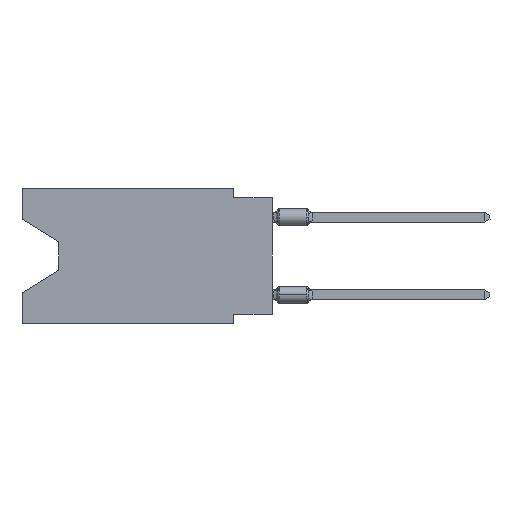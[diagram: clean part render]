
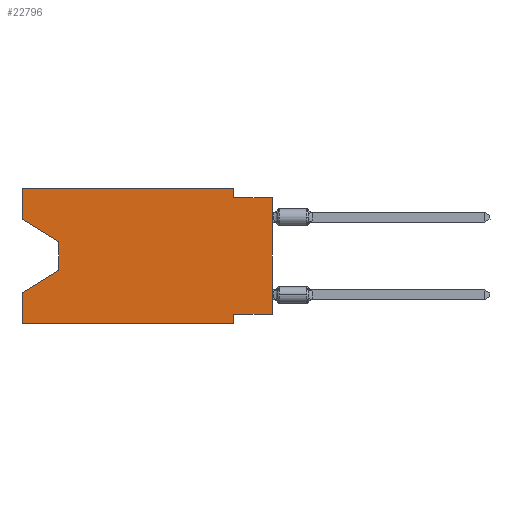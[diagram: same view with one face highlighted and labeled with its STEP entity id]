
A CAD part, left-side view. The second image highlights one B-rep face of the part: STEP entity #22796.
In plain terms, the highlighted planar face has unit normal (-1, 0, 0).
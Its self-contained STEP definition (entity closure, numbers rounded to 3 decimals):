
#113 = CARTESIAN_POINT ( 'NONE',  ( 0., 16.383, 0. ) ) ;
#532 = VERTEX_POINT ( 'NONE', #19451 ) ;
#1204 = EDGE_CURVE ( 'NONE', #12991, #24215, #21346, .T. ) ;
#1276 = VECTOR ( 'NONE', #21200, 1000. ) ;
#1779 = CARTESIAN_POINT ( 'NONE',  ( 0., 16.383, -8.89 ) ) ;
#1817 = CARTESIAN_POINT ( 'NONE',  ( 0., 13.97, -3.505 ) ) ;
#2605 = LINE ( 'NONE', #20838, #26267 ) ;
#3109 = VERTEX_POINT ( 'NONE', #23534 ) ;
#3121 = VERTEX_POINT ( 'NONE', #30328 ) ;
#3627 = EDGE_CURVE ( 'NONE', #6802, #29705, #21899, .T. ) ;
#3643 = CARTESIAN_POINT ( 'NONE',  ( 0., 16.383, -6.852 ) ) ;
#3694 = VECTOR ( 'NONE', #18195, 1000. ) ;
#3832 = LINE ( 'NONE', #1817, #3694 ) ;
#4683 = CARTESIAN_POINT ( 'NONE',  ( 0., 0., 0. ) ) ;
#4834 = VECTOR ( 'NONE', #29973, 1000. ) ;
#5129 = VERTEX_POINT ( 'NONE', #8794 ) ;
#5276 = CARTESIAN_POINT ( 'NONE',  ( 0., 0., -8.255 ) ) ;
#6111 = FACE_OUTER_BOUND ( 'NONE', #15059, .T. ) ;
#6137 = CARTESIAN_POINT ( 'NONE',  ( 0., 13.97, -5.385 ) ) ;
#6257 = VECTOR ( 'NONE', #30333, 1000. ) ;
#6549 = VERTEX_POINT ( 'NONE', #25130 ) ;
#6802 = VERTEX_POINT ( 'NONE', #9281 ) ;
#7530 = DIRECTION ( 'NONE',  ( 0., 0., -1. ) ) ;
#7658 = VERTEX_POINT ( 'NONE', #25699 ) ;
#8290 = DIRECTION ( 'NONE',  ( 0., 0.855, -0.519 ) ) ;
#8420 = EDGE_CURVE ( 'NONE', #3109, #6549, #2605, .T. ) ;
#8794 = CARTESIAN_POINT ( 'NONE',  ( 0., 0., -0.635 ) ) ;
#9281 = CARTESIAN_POINT ( 'NONE',  ( 0., 2.54, 0. ) ) ;
#9352 = ORIENTED_EDGE ( 'NONE', *, *, #14881, .F. ) ;
#9777 = ORIENTED_EDGE ( 'NONE', *, *, #25870, .T. ) ;
#10155 = CARTESIAN_POINT ( 'NONE',  ( 0., 2.54, 0. ) ) ;
#10588 = CARTESIAN_POINT ( 'NONE',  ( 0., 16.383, 0. ) ) ;
#11511 = ORIENTED_EDGE ( 'NONE', *, *, #15652, .T. ) ;
#12054 = LINE ( 'NONE', #20872, #18426 ) ;
#12399 = LINE ( 'NONE', #23833, #14665 ) ;
#12660 = EDGE_CURVE ( 'NONE', #13070, #26617, #17886, .T. ) ;
#12991 = VERTEX_POINT ( 'NONE', #22790 ) ;
#13070 = VERTEX_POINT ( 'NONE', #1779 ) ;
#13263 = CARTESIAN_POINT ( 'NONE',  ( 0., 16.383, 0. ) ) ;
#13536 = PLANE ( 'NONE',  #21171 ) ;
#14126 = CARTESIAN_POINT ( 'NONE',  ( 0., 16.383, 0. ) ) ;
#14665 = VECTOR ( 'NONE', #14713, 1000. ) ;
#14713 = DIRECTION ( 'NONE',  ( 0., -1., 0. ) ) ;
#14881 = EDGE_CURVE ( 'NONE', #29705, #5129, #12054, .T. ) ;
#15059 = EDGE_LOOP ( 'NONE', ( #28800, #29472, #11511, #16471, #29286, #18075, #29370, #9777, #9352, #29704, #25411, #24795 ) ) ;
#15119 = CARTESIAN_POINT ( 'NONE',  ( 0., 2.54, -8.89 ) ) ;
#15652 = EDGE_CURVE ( 'NONE', #7658, #26617, #27285, .T. ) ;
#15930 = LINE ( 'NONE', #113, #4834 ) ;
#16471 = ORIENTED_EDGE ( 'NONE', *, *, #12660, .F. ) ;
#16947 = EDGE_CURVE ( 'NONE', #6549, #7658, #3832, .T. ) ;
#17379 = EDGE_CURVE ( 'NONE', #3109, #532, #23243, .T. ) ;
#17431 = LINE ( 'NONE', #15119, #27111 ) ;
#17610 = VECTOR ( 'NONE', #8290, 1000. ) ;
#17886 = LINE ( 'NONE', #13263, #26688 ) ;
#18075 = ORIENTED_EDGE ( 'NONE', *, *, #26259, .F. ) ;
#18195 = DIRECTION ( 'NONE',  ( 0., 0., -1. ) ) ;
#18426 = VECTOR ( 'NONE', #23200, 1000. ) ;
#19451 = CARTESIAN_POINT ( 'NONE',  ( 0., 16.383, 0. ) ) ;
#19644 = VECTOR ( 'NONE', #7530, 1000. ) ;
#19900 = DIRECTION ( 'NONE',  ( 0., 0., -1. ) ) ;
#20011 = DIRECTION ( 'NONE',  ( 1., 0., 0. ) ) ;
#20838 = CARTESIAN_POINT ( 'NONE',  ( 0., 16.383, -2.038 ) ) ;
#20872 = CARTESIAN_POINT ( 'NONE',  ( 0., 0., -0.635 ) ) ;
#20986 = DIRECTION ( 'NONE',  ( 0., -0.855, -0.519 ) ) ;
#21171 = AXIS2_PLACEMENT_3D ( 'NONE', #10588, #20011, #30050 ) ;
#21200 = DIRECTION ( 'NONE',  ( 0., 1., 0. ) ) ;
#21209 = LINE ( 'NONE', #4683, #25578 ) ;
#21346 = LINE ( 'NONE', #5276, #1276 ) ;
#21899 = LINE ( 'NONE', #10155, #19644 ) ;
#22790 = CARTESIAN_POINT ( 'NONE',  ( 0., 0., -8.255 ) ) ;
#22796 = ADVANCED_FACE ( 'NONE', ( #6111 ), #13536, .F. ) ;
#23200 = DIRECTION ( 'NONE',  ( 0., -1., 0. ) ) ;
#23243 = LINE ( 'NONE', #14126, #6257 ) ;
#23534 = CARTESIAN_POINT ( 'NONE',  ( 0., 16.383, -2.038 ) ) ;
#23686 = DIRECTION ( 'NONE',  ( 0., 0., 1. ) ) ;
#23775 = EDGE_CURVE ( 'NONE', #532, #6802, #15930, .T. ) ;
#23833 = CARTESIAN_POINT ( 'NONE',  ( 0., 16.383, -8.89 ) ) ;
#24215 = VERTEX_POINT ( 'NONE', #28341 ) ;
#24795 = ORIENTED_EDGE ( 'NONE', *, *, #17379, .F. ) ;
#25130 = CARTESIAN_POINT ( 'NONE',  ( 0., 13.97, -3.505 ) ) ;
#25411 = ORIENTED_EDGE ( 'NONE', *, *, #23775, .F. ) ;
#25578 = VECTOR ( 'NONE', #23686, 1000. ) ;
#25699 = CARTESIAN_POINT ( 'NONE',  ( 0., 13.97, -5.385 ) ) ;
#25870 = EDGE_CURVE ( 'NONE', #12991, #5129, #21209, .T. ) ;
#26259 = EDGE_CURVE ( 'NONE', #24215, #3121, #17431, .T. ) ;
#26267 = VECTOR ( 'NONE', #20986, 1000. ) ;
#26617 = VERTEX_POINT ( 'NONE', #3643 ) ;
#26688 = VECTOR ( 'NONE', #27758, 1000. ) ;
#27111 = VECTOR ( 'NONE', #19900, 1000. ) ;
#27285 = LINE ( 'NONE', #6137, #17610 ) ;
#27758 = DIRECTION ( 'NONE',  ( 0., 0., 1. ) ) ;
#28341 = CARTESIAN_POINT ( 'NONE',  ( 0., 2.54, -8.255 ) ) ;
#28767 = CARTESIAN_POINT ( 'NONE',  ( 0., 2.54, -0.635 ) ) ;
#28800 = ORIENTED_EDGE ( 'NONE', *, *, #8420, .T. ) ;
#29286 = ORIENTED_EDGE ( 'NONE', *, *, #29789, .T. ) ;
#29370 = ORIENTED_EDGE ( 'NONE', *, *, #1204, .F. ) ;
#29472 = ORIENTED_EDGE ( 'NONE', *, *, #16947, .T. ) ;
#29704 = ORIENTED_EDGE ( 'NONE', *, *, #3627, .F. ) ;
#29705 = VERTEX_POINT ( 'NONE', #28767 ) ;
#29789 = EDGE_CURVE ( 'NONE', #13070, #3121, #12399, .T. ) ;
#29973 = DIRECTION ( 'NONE',  ( 0., -1., 0. ) ) ;
#30050 = DIRECTION ( 'NONE',  ( 0., 0., -1. ) ) ;
#30328 = CARTESIAN_POINT ( 'NONE',  ( 0., 2.54, -8.89 ) ) ;
#30333 = DIRECTION ( 'NONE',  ( 0., 0., 1. ) ) ;
